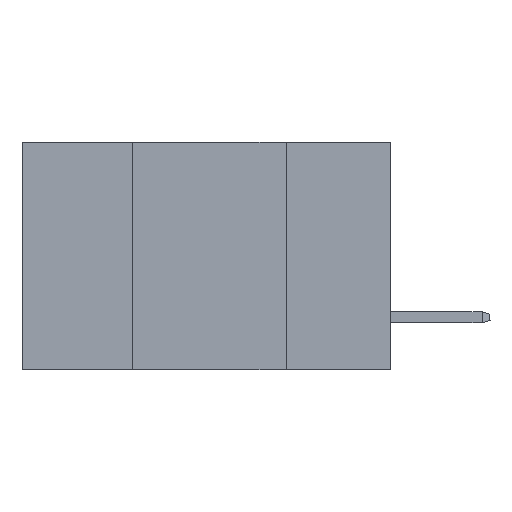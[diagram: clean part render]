
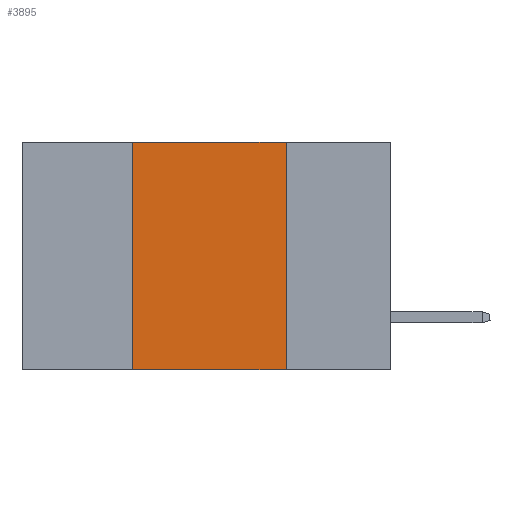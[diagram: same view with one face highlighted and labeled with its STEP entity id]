
A CAD part, left-side view. The second image highlights one B-rep face of the part: STEP entity #3895.
In plain terms, the highlighted planar face has unit normal (-1, 0, 0).
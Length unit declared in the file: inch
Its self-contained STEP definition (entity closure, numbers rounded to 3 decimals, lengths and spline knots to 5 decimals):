
#2512 = VECTOR ( 'NONE', #3253, 39.37008 ) ;
#3253 = DIRECTION ( 'NONE',  ( 0., -1., 0. ) ) ;
#3895 = ADVANCED_FACE ( 'NONE', ( #30537 ), #31731, .F. ) ;
#4233 = CARTESIAN_POINT ( 'NONE',  ( 0., 0.42, 0. ) ) ;
#4361 = ORIENTED_EDGE ( 'NONE', *, *, #19937, .T. ) ;
#5651 = LINE ( 'NONE', #36461, #30223 ) ;
#9524 = VECTOR ( 'NONE', #11462, 39.37008 ) ;
#9704 = CARTESIAN_POINT ( 'NONE',  ( 0., 0.6, -0.37 ) ) ;
#9953 = DIRECTION ( 'NONE',  ( 0., 0., 1. ) ) ;
#11061 = DIRECTION ( 'NONE',  ( 1., 0., 0. ) ) ;
#11462 = DIRECTION ( 'NONE',  ( 0., 0., -1. ) ) ;
#12606 = DIRECTION ( 'NONE',  ( 0., 0., -1. ) ) ;
#12923 = DIRECTION ( 'NONE',  ( 0., -1., 0. ) ) ;
#15374 = CARTESIAN_POINT ( 'NONE',  ( 0., 0.42, 0. ) ) ;
#16030 = VERTEX_POINT ( 'NONE', #15374 ) ;
#16060 = VERTEX_POINT ( 'NONE', #19681 ) ;
#16625 = AXIS2_PLACEMENT_3D ( 'NONE', #25700, #11061, #12606 ) ;
#17280 = ORIENTED_EDGE ( 'NONE', *, *, #36057, .F. ) ;
#17540 = EDGE_CURVE ( 'NONE', #38285, #16030, #22785, .T. ) ;
#18037 = LINE ( 'NONE', #22152, #9524 ) ;
#19681 = CARTESIAN_POINT ( 'NONE',  ( 0., 0.17, -0.37 ) ) ;
#19937 = EDGE_CURVE ( 'NONE', #38285, #16060, #36135, .T. ) ;
#20857 = EDGE_CURVE ( 'NONE', #21103, #16060, #18037, .T. ) ;
#21103 = VERTEX_POINT ( 'NONE', #34059 ) ;
#22152 = CARTESIAN_POINT ( 'NONE',  ( 0., 0.17, 0. ) ) ;
#22785 = LINE ( 'NONE', #4233, #30330 ) ;
#25700 = CARTESIAN_POINT ( 'NONE',  ( 0., 0.6, 0. ) ) ;
#30223 = VECTOR ( 'NONE', #12923, 39.37008 ) ;
#30330 = VECTOR ( 'NONE', #9953, 39.37008 ) ;
#30537 = FACE_OUTER_BOUND ( 'NONE', #31570, .T. ) ;
#31570 = EDGE_LOOP ( 'NONE', ( #38182, #17280, #41537, #4361 ) ) ;
#31731 = PLANE ( 'NONE',  #16625 ) ;
#34059 = CARTESIAN_POINT ( 'NONE',  ( 0., 0.17, 0. ) ) ;
#35781 = CARTESIAN_POINT ( 'NONE',  ( 0., 0.42, -0.37 ) ) ;
#36057 = EDGE_CURVE ( 'NONE', #16030, #21103, #5651, .T. ) ;
#36135 = LINE ( 'NONE', #9704, #2512 ) ;
#36461 = CARTESIAN_POINT ( 'NONE',  ( 0., 0.6, 0. ) ) ;
#38182 = ORIENTED_EDGE ( 'NONE', *, *, #20857, .F. ) ;
#38285 = VERTEX_POINT ( 'NONE', #35781 ) ;
#41537 = ORIENTED_EDGE ( 'NONE', *, *, #17540, .F. ) ;
